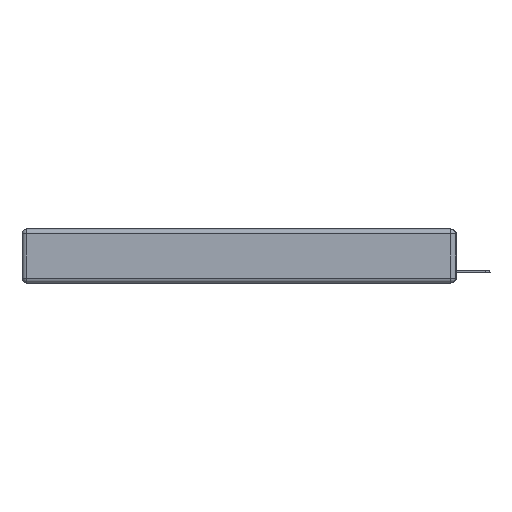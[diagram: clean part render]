
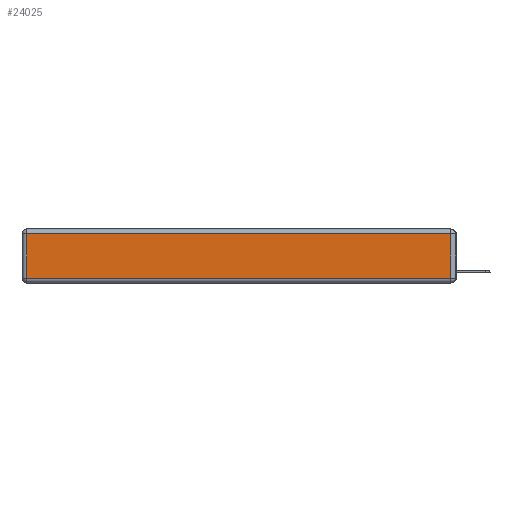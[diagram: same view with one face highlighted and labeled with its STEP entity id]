
A CAD part, left-side view. The second image highlights one B-rep face of the part: STEP entity #24025.
In plain terms, the highlighted planar face has unit normal (-1, 0, 0).
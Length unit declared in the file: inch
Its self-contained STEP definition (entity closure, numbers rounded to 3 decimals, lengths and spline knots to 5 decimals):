
#751 = EDGE_CURVE ( 'NONE', #4482, #2330, #9201, .T. ) ;
#1483 = CARTESIAN_POINT ( 'NONE',  ( 0., 0.03, -0.03 ) ) ;
#2330 = VERTEX_POINT ( 'NONE', #1483 ) ;
#2930 = CARTESIAN_POINT ( 'NONE',  ( 0., 2.75, -0.03 ) ) ;
#4482 = VERTEX_POINT ( 'NONE', #20316 ) ;
#4750 = ORIENTED_EDGE ( 'NONE', *, *, #19972, .T. ) ;
#6083 = CARTESIAN_POINT ( 'NONE',  ( 0., 2.72, -0.03 ) ) ;
#6385 = PLANE ( 'NONE',  #26290 ) ;
#6401 = ORIENTED_EDGE ( 'NONE', *, *, #18496, .T. ) ;
#6985 = ORIENTED_EDGE ( 'NONE', *, *, #16744, .T. ) ;
#7961 = CARTESIAN_POINT ( 'NONE',  ( 0., 2.72, -0.343 ) ) ;
#8516 = DIRECTION ( 'NONE',  ( 0., 0., 1. ) ) ;
#8657 = FACE_OUTER_BOUND ( 'NONE', #12228, .T. ) ;
#9201 = LINE ( 'NONE', #11180, #18417 ) ;
#9781 = DIRECTION ( 'NONE',  ( 0., -1., 0. ) ) ;
#10092 = LINE ( 'NONE', #7961, #14464 ) ;
#10504 = DIRECTION ( 'NONE',  ( -1., 0., 0. ) ) ;
#11180 = CARTESIAN_POINT ( 'NONE',  ( 0., 0.03, -0.343 ) ) ;
#12228 = EDGE_LOOP ( 'NONE', ( #4750, #12419, #6985, #6401 ) ) ;
#12419 = ORIENTED_EDGE ( 'NONE', *, *, #751, .T. ) ;
#13610 = CARTESIAN_POINT ( 'NONE',  ( 0., 2.72, -0.313 ) ) ;
#14464 = VECTOR ( 'NONE', #18554, 39.37008 ) ;
#16744 = EDGE_CURVE ( 'NONE', #2330, #18849, #22796, .T. ) ;
#17058 = VECTOR ( 'NONE', #24489, 39.37008 ) ;
#17809 = DIRECTION ( 'NONE',  ( 0., 0., 1. ) ) ;
#18112 = CARTESIAN_POINT ( 'NONE',  ( 0., 0., -0.313 ) ) ;
#18417 = VECTOR ( 'NONE', #17809, 39.37008 ) ;
#18496 = EDGE_CURVE ( 'NONE', #18849, #25809, #10092, .T. ) ;
#18554 = DIRECTION ( 'NONE',  ( 0., 0., -1. ) ) ;
#18849 = VERTEX_POINT ( 'NONE', #6083 ) ;
#19027 = VECTOR ( 'NONE', #9781, 39.37008 ) ;
#19672 = LINE ( 'NONE', #18112, #19027 ) ;
#19972 = EDGE_CURVE ( 'NONE', #25809, #4482, #19672, .T. ) ;
#20316 = CARTESIAN_POINT ( 'NONE',  ( 0., 0.03, -0.313 ) ) ;
#22796 = LINE ( 'NONE', #2930, #17058 ) ;
#24025 = ADVANCED_FACE ( 'NONE', ( #8657 ), #6385, .T. ) ;
#24489 = DIRECTION ( 'NONE',  ( 0., 1., 0. ) ) ;
#25809 = VERTEX_POINT ( 'NONE', #13610 ) ;
#26290 = AXIS2_PLACEMENT_3D ( 'NONE', #27811, #10504, #8516 ) ;
#27811 = CARTESIAN_POINT ( 'NONE',  ( 0., 0., -0.343 ) ) ;
